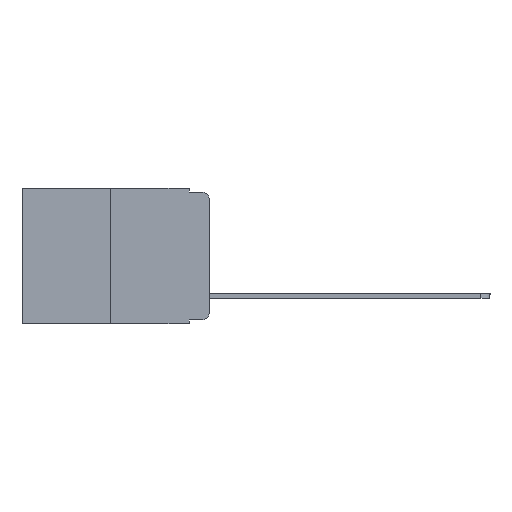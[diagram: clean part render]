
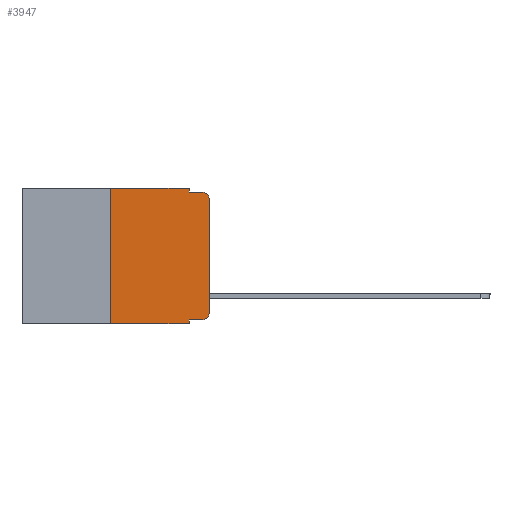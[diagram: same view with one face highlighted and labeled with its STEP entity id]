
A CAD part, left-side view. The second image highlights one B-rep face of the part: STEP entity #3947.
In plain terms, the highlighted planar face has unit normal (-1, 0, 0).
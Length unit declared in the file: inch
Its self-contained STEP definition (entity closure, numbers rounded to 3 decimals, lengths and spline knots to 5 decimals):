
#213 = DIRECTION ( 'NONE',  ( 0., 0., -1. ) ) ;
#792 = EDGE_CURVE ( 'NONE', #8665, #14842, #10184, .T. ) ;
#1415 = DIRECTION ( 'NONE',  ( 0., 0., 1. ) ) ;
#1468 = VERTEX_POINT ( 'NONE', #9821 ) ;
#1625 = VECTOR ( 'NONE', #2900, 39.37008 ) ;
#1673 = ORIENTED_EDGE ( 'NONE', *, *, #10820, .F. ) ;
#1809 = EDGE_CURVE ( 'NONE', #5736, #7597, #13218, .T. ) ;
#2657 = DIRECTION ( 'NONE',  ( -1., 0., 0. ) ) ;
#2900 = DIRECTION ( 'NONE',  ( 0., -1., 0. ) ) ;
#2954 = VERTEX_POINT ( 'NONE', #14444 ) ;
#3034 = ORIENTED_EDGE ( 'NONE', *, *, #792, .F. ) ;
#3830 = EDGE_CURVE ( 'NONE', #1468, #15049, #9643, .T. ) ;
#3892 = ORIENTED_EDGE ( 'NONE', *, *, #4742, .F. ) ;
#3947 = ADVANCED_FACE ( 'NONE', ( #9261 ), #9344, .F. ) ;
#4263 = CARTESIAN_POINT ( 'NONE',  ( 0., 0.051, -0.333 ) ) ;
#4290 = VECTOR ( 'NONE', #4434, 39.37008 ) ;
#4360 = CARTESIAN_POINT ( 'NONE',  ( 0., 0.051, 0. ) ) ;
#4434 = DIRECTION ( 'NONE',  ( 0., 0., -1. ) ) ;
#4485 = CARTESIAN_POINT ( 'NONE',  ( 0., 0.473, 0. ) ) ;
#4494 = EDGE_CURVE ( 'NONE', #10575, #8816, #5800, .T. ) ;
#4669 = ORIENTED_EDGE ( 'NONE', *, *, #1809, .T. ) ;
#4742 = EDGE_CURVE ( 'NONE', #10575, #8665, #8128, .T. ) ;
#5072 = VECTOR ( 'NONE', #10345, 39.37008 ) ;
#5256 = ORIENTED_EDGE ( 'NONE', *, *, #4494, .T. ) ;
#5470 = CARTESIAN_POINT ( 'NONE',  ( 0., 0.051, -0.01 ) ) ;
#5736 = VERTEX_POINT ( 'NONE', #12906 ) ;
#5800 = LINE ( 'NONE', #14969, #8532 ) ;
#5894 = AXIS2_PLACEMENT_3D ( 'NONE', #15492, #10436, #11145 ) ;
#6462 = EDGE_CURVE ( 'NONE', #2954, #5736, #11728, .T. ) ;
#6999 = DIRECTION ( 'NONE',  ( 1., 0., 0. ) ) ;
#7090 = EDGE_LOOP ( 'NONE', ( #12689, #12331, #16072, #1673, #3034, #3892, #5256, #13141, #10675, #4669 ) ) ;
#7143 = CARTESIAN_POINT ( 'NONE',  ( 0., 0.051, -0.343 ) ) ;
#7361 = DIRECTION ( 'NONE',  ( 0., 0., -1. ) ) ;
#7597 = VERTEX_POINT ( 'NONE', #16152 ) ;
#7780 = VECTOR ( 'NONE', #10302, 39.37008 ) ;
#8128 = LINE ( 'NONE', #15632, #11495 ) ;
#8314 = CARTESIAN_POINT ( 'NONE',  ( 0., 0., 0. ) ) ;
#8532 = VECTOR ( 'NONE', #10914, 39.37008 ) ;
#8631 = LINE ( 'NONE', #8957, #8987 ) ;
#8665 = VERTEX_POINT ( 'NONE', #12665 ) ;
#8795 = CARTESIAN_POINT ( 'NONE',  ( 0., 0.25, -0.343 ) ) ;
#8813 = CARTESIAN_POINT ( 'NONE',  ( 0., 0.051, 0. ) ) ;
#8816 = VERTEX_POINT ( 'NONE', #7143 ) ;
#8957 = CARTESIAN_POINT ( 'NONE',  ( 0., 0.051, 0. ) ) ;
#8987 = VECTOR ( 'NONE', #7361, 39.37008 ) ;
#9261 = FACE_OUTER_BOUND ( 'NONE', #7090, .T. ) ;
#9344 = PLANE ( 'NONE',  #14209 ) ;
#9421 = LINE ( 'NONE', #8314, #11547 ) ;
#9643 = CIRCLE ( 'NONE', #5894, 0.02 ) ;
#9816 = CARTESIAN_POINT ( 'NONE',  ( 0., 0.02, -0.01 ) ) ;
#9821 = CARTESIAN_POINT ( 'NONE',  ( 0., 0., -0.03 ) ) ;
#10184 = LINE ( 'NONE', #12644, #5072 ) ;
#10302 = DIRECTION ( 'NONE',  ( 0., -1., 0. ) ) ;
#10345 = DIRECTION ( 'NONE',  ( 0., -1., 0. ) ) ;
#10436 = DIRECTION ( 'NONE',  ( -1., 0., 0. ) ) ;
#10575 = VERTEX_POINT ( 'NONE', #8795 ) ;
#10675 = ORIENTED_EDGE ( 'NONE', *, *, #6462, .T. ) ;
#10820 = EDGE_CURVE ( 'NONE', #14842, #14592, #13434, .T. ) ;
#10914 = DIRECTION ( 'NONE',  ( 0., -1., 0. ) ) ;
#11145 = DIRECTION ( 'NONE',  ( 0., 0., -1. ) ) ;
#11495 = VECTOR ( 'NONE', #1415, 39.37008 ) ;
#11547 = VECTOR ( 'NONE', #13305, 39.37008 ) ;
#11604 = EDGE_CURVE ( 'NONE', #7597, #1468, #9421, .T. ) ;
#11728 = LINE ( 'NONE', #4263, #1625 ) ;
#11730 = LINE ( 'NONE', #16598, #7780 ) ;
#11784 = DIRECTION ( 'NONE',  ( 0., 0., -1. ) ) ;
#12331 = ORIENTED_EDGE ( 'NONE', *, *, #3830, .T. ) ;
#12644 = CARTESIAN_POINT ( 'NONE',  ( 0., 0.473, 0. ) ) ;
#12665 = CARTESIAN_POINT ( 'NONE',  ( 0., 0.25, 0. ) ) ;
#12689 = ORIENTED_EDGE ( 'NONE', *, *, #11604, .T. ) ;
#12906 = CARTESIAN_POINT ( 'NONE',  ( 0., 0.02, -0.333 ) ) ;
#13141 = ORIENTED_EDGE ( 'NONE', *, *, #16460, .F. ) ;
#13218 = CIRCLE ( 'NONE', #14283, 0.02 ) ;
#13305 = DIRECTION ( 'NONE',  ( 0., 0., 1. ) ) ;
#13434 = LINE ( 'NONE', #4360, #4290 ) ;
#13529 = EDGE_CURVE ( 'NONE', #14592, #15049, #11730, .T. ) ;
#14183 = CARTESIAN_POINT ( 'NONE',  ( 0., 0.02, -0.313 ) ) ;
#14209 = AXIS2_PLACEMENT_3D ( 'NONE', #4485, #6999, #11784 ) ;
#14283 = AXIS2_PLACEMENT_3D ( 'NONE', #14183, #2657, #213 ) ;
#14444 = CARTESIAN_POINT ( 'NONE',  ( 0., 0.051, -0.333 ) ) ;
#14592 = VERTEX_POINT ( 'NONE', #5470 ) ;
#14842 = VERTEX_POINT ( 'NONE', #8813 ) ;
#14969 = CARTESIAN_POINT ( 'NONE',  ( 0., 0.473, -0.343 ) ) ;
#15049 = VERTEX_POINT ( 'NONE', #9816 ) ;
#15492 = CARTESIAN_POINT ( 'NONE',  ( 0., 0.02, -0.03 ) ) ;
#15632 = CARTESIAN_POINT ( 'NONE',  ( 0., 0.25, 0. ) ) ;
#16072 = ORIENTED_EDGE ( 'NONE', *, *, #13529, .F. ) ;
#16152 = CARTESIAN_POINT ( 'NONE',  ( 0., 0., -0.313 ) ) ;
#16460 = EDGE_CURVE ( 'NONE', #2954, #8816, #8631, .T. ) ;
#16598 = CARTESIAN_POINT ( 'NONE',  ( 0., 0.051, -0.01 ) ) ;
